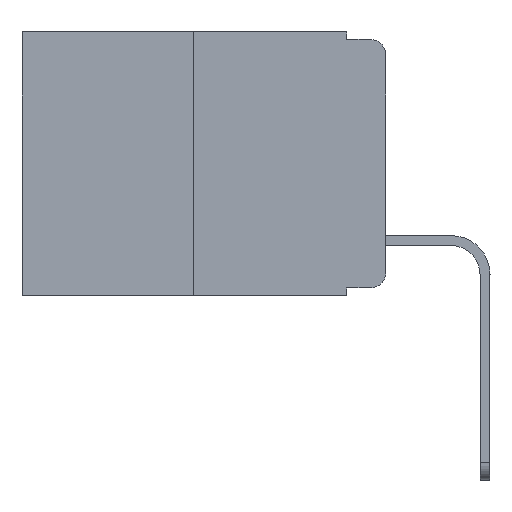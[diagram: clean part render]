
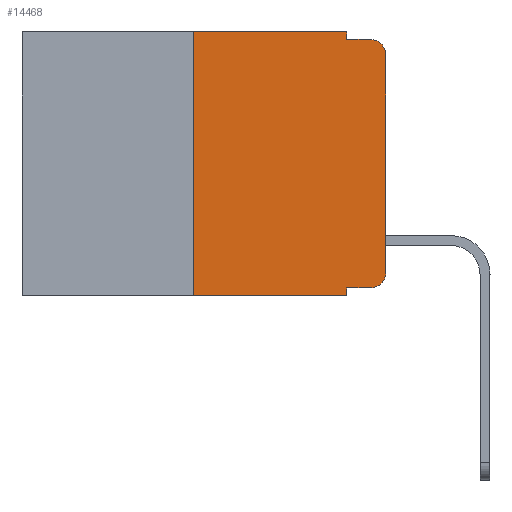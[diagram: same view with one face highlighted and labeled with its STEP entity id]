
A CAD part, left-side view. The second image highlights one B-rep face of the part: STEP entity #14468.
In plain terms, the highlighted planar face has unit normal (-1, 0, 0).
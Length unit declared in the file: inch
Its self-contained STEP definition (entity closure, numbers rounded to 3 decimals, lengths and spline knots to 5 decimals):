
#144 = ORIENTED_EDGE ( 'NONE', *, *, #10706, .T. ) ;
#157 = CARTESIAN_POINT ( 'NONE',  ( 0., 0., -0.313 ) ) ;
#367 = CARTESIAN_POINT ( 'NONE',  ( 0., 0., -0.03 ) ) ;
#524 = CARTESIAN_POINT ( 'NONE',  ( 0., 0.473, 0. ) ) ;
#916 = CARTESIAN_POINT ( 'NONE',  ( 0., 0.473, 0. ) ) ;
#1170 = DIRECTION ( 'NONE',  ( 0., 0., 1. ) ) ;
#1309 = DIRECTION ( 'NONE',  ( 0., 0., 1. ) ) ;
#1382 = DIRECTION ( 'NONE',  ( 0., -1., 0. ) ) ;
#1635 = ORIENTED_EDGE ( 'NONE', *, *, #14561, .T. ) ;
#1694 = LINE ( 'NONE', #11184, #12443 ) ;
#2512 = ORIENTED_EDGE ( 'NONE', *, *, #7149, .F. ) ;
#2814 = CARTESIAN_POINT ( 'NONE',  ( 0., 0.02, -0.333 ) ) ;
#4023 = DIRECTION ( 'NONE',  ( 0., 0., -1. ) ) ;
#4168 = ORIENTED_EDGE ( 'NONE', *, *, #17663, .T. ) ;
#4465 = VERTEX_POINT ( 'NONE', #9429 ) ;
#4668 = VERTEX_POINT ( 'NONE', #13275 ) ;
#4983 = LINE ( 'NONE', #524, #14639 ) ;
#5179 = LINE ( 'NONE', #18807, #7021 ) ;
#5312 = DIRECTION ( 'NONE',  ( -1., 0., 0. ) ) ;
#5315 = CARTESIAN_POINT ( 'NONE',  ( 0., 0.25, 0. ) ) ;
#6050 = VECTOR ( 'NONE', #17682, 39.37008 ) ;
#6185 = EDGE_CURVE ( 'NONE', #9084, #14010, #6859, .T. ) ;
#6526 = DIRECTION ( 'NONE',  ( 0., 0., -1. ) ) ;
#6647 = DIRECTION ( 'NONE',  ( 0., 0., -1. ) ) ;
#6849 = CARTESIAN_POINT ( 'NONE',  ( 0., 0.051, 0. ) ) ;
#6859 = LINE ( 'NONE', #6849, #18084 ) ;
#6869 = EDGE_CURVE ( 'NONE', #17878, #16423, #10510, .T. ) ;
#6873 = CARTESIAN_POINT ( 'NONE',  ( 0., 0.051, 0. ) ) ;
#7005 = CIRCLE ( 'NONE', #7490, 0.02 ) ;
#7021 = VECTOR ( 'NONE', #1382, 39.37008 ) ;
#7041 = VECTOR ( 'NONE', #18719, 39.37008 ) ;
#7119 = CARTESIAN_POINT ( 'NONE',  ( 0., 0.051, -0.333 ) ) ;
#7149 = EDGE_CURVE ( 'NONE', #16423, #7718, #4983, .T. ) ;
#7486 = DIRECTION ( 'NONE',  ( 0., 0., -1. ) ) ;
#7490 = AXIS2_PLACEMENT_3D ( 'NONE', #18591, #9837, #7486 ) ;
#7718 = VERTEX_POINT ( 'NONE', #9291 ) ;
#8115 = AXIS2_PLACEMENT_3D ( 'NONE', #916, #15548, #4023 ) ;
#8531 = CARTESIAN_POINT ( 'NONE',  ( 0., 0.473, -0.343 ) ) ;
#8671 = EDGE_LOOP ( 'NONE', ( #144, #4168, #10536, #17228, #2512, #8822, #17839, #16863, #10132, #1635 ) ) ;
#8822 = ORIENTED_EDGE ( 'NONE', *, *, #6869, .F. ) ;
#9084 = VERTEX_POINT ( 'NONE', #7119 ) ;
#9291 = CARTESIAN_POINT ( 'NONE',  ( 0., 0.051, 0. ) ) ;
#9305 = VECTOR ( 'NONE', #18766, 39.37008 ) ;
#9429 = CARTESIAN_POINT ( 'NONE',  ( 0., 0.051, -0.01 ) ) ;
#9511 = LINE ( 'NONE', #13382, #6050 ) ;
#9837 = DIRECTION ( 'NONE',  ( -1., 0., 0. ) ) ;
#9910 = CARTESIAN_POINT ( 'NONE',  ( 0., 0.25, 0. ) ) ;
#10132 = ORIENTED_EDGE ( 'NONE', *, *, #14671, .T. ) ;
#10510 = LINE ( 'NONE', #9910, #16469 ) ;
#10536 = ORIENTED_EDGE ( 'NONE', *, *, #17131, .F. ) ;
#10706 = EDGE_CURVE ( 'NONE', #12448, #11825, #1694, .T. ) ;
#11184 = CARTESIAN_POINT ( 'NONE',  ( 0., 0., 0. ) ) ;
#11299 = CARTESIAN_POINT ( 'NONE',  ( 0., 0.25, -0.343 ) ) ;
#11825 = VERTEX_POINT ( 'NONE', #367 ) ;
#12388 = CARTESIAN_POINT ( 'NONE',  ( 0., 0.02, -0.03 ) ) ;
#12443 = VECTOR ( 'NONE', #1170, 39.37008 ) ;
#12448 = VERTEX_POINT ( 'NONE', #157 ) ;
#12790 = EDGE_CURVE ( 'NONE', #7718, #4465, #17605, .T. ) ;
#13275 = CARTESIAN_POINT ( 'NONE',  ( 0., 0.02, -0.01 ) ) ;
#13382 = CARTESIAN_POINT ( 'NONE',  ( 0., 0.051, -0.333 ) ) ;
#14010 = VERTEX_POINT ( 'NONE', #14539 ) ;
#14372 = LINE ( 'NONE', #8531, #9305 ) ;
#14376 = FACE_OUTER_BOUND ( 'NONE', #8671, .T. ) ;
#14468 = ADVANCED_FACE ( 'NONE', ( #14376 ), #16950, .F. ) ;
#14539 = CARTESIAN_POINT ( 'NONE',  ( 0., 0.051, -0.343 ) ) ;
#14561 = EDGE_CURVE ( 'NONE', #18516, #12448, #7005, .T. ) ;
#14639 = VECTOR ( 'NONE', #14903, 39.37008 ) ;
#14671 = EDGE_CURVE ( 'NONE', #9084, #18516, #9511, .T. ) ;
#14903 = DIRECTION ( 'NONE',  ( 0., -1., 0. ) ) ;
#15548 = DIRECTION ( 'NONE',  ( 1., 0., 0. ) ) ;
#16423 = VERTEX_POINT ( 'NONE', #5315 ) ;
#16469 = VECTOR ( 'NONE', #1309, 39.37008 ) ;
#16863 = ORIENTED_EDGE ( 'NONE', *, *, #6185, .F. ) ;
#16950 = PLANE ( 'NONE',  #8115 ) ;
#17131 = EDGE_CURVE ( 'NONE', #4465, #4668, #5179, .T. ) ;
#17228 = ORIENTED_EDGE ( 'NONE', *, *, #12790, .F. ) ;
#17329 = CIRCLE ( 'NONE', #18195, 0.02 ) ;
#17492 = EDGE_CURVE ( 'NONE', #17878, #14010, #14372, .T. ) ;
#17605 = LINE ( 'NONE', #6873, #7041 ) ;
#17663 = EDGE_CURVE ( 'NONE', #11825, #4668, #17329, .T. ) ;
#17682 = DIRECTION ( 'NONE',  ( 0., -1., 0. ) ) ;
#17839 = ORIENTED_EDGE ( 'NONE', *, *, #17492, .T. ) ;
#17878 = VERTEX_POINT ( 'NONE', #11299 ) ;
#18084 = VECTOR ( 'NONE', #6647, 39.37008 ) ;
#18195 = AXIS2_PLACEMENT_3D ( 'NONE', #12388, #5312, #6526 ) ;
#18516 = VERTEX_POINT ( 'NONE', #2814 ) ;
#18591 = CARTESIAN_POINT ( 'NONE',  ( 0., 0.02, -0.313 ) ) ;
#18719 = DIRECTION ( 'NONE',  ( 0., 0., -1. ) ) ;
#18766 = DIRECTION ( 'NONE',  ( 0., -1., 0. ) ) ;
#18807 = CARTESIAN_POINT ( 'NONE',  ( 0., 0.051, -0.01 ) ) ;
